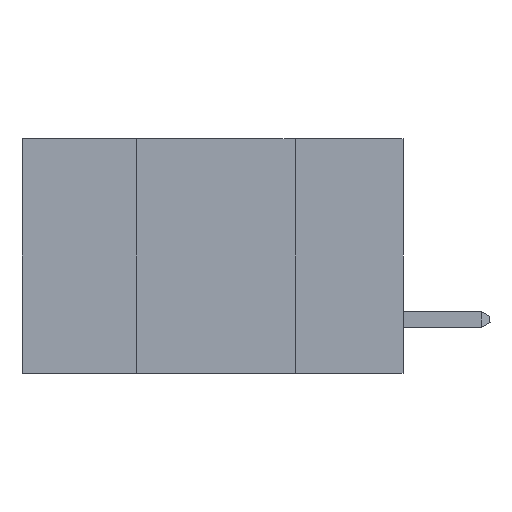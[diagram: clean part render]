
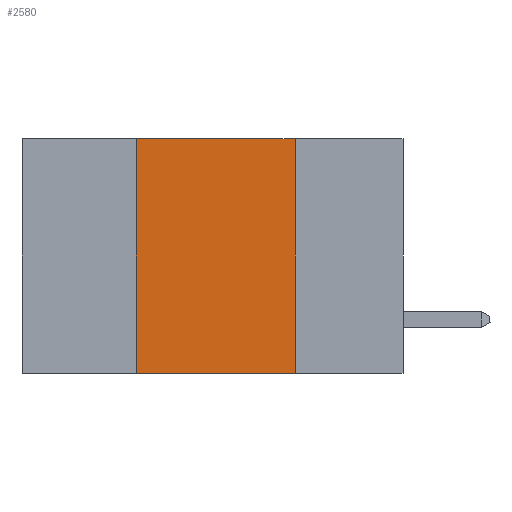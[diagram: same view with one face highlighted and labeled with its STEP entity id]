
A CAD part, left-side view. The second image highlights one B-rep face of the part: STEP entity #2580.
In plain terms, the highlighted planar face has unit normal (-1, 0, 0).
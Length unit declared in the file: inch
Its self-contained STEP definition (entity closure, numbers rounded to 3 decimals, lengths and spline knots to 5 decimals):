
#1754 = VERTEX_POINT ( 'NONE', #9888 ) ;
#2580 = ADVANCED_FACE ( 'NONE', ( #19786 ), #27750, .F. ) ;
#2932 = LINE ( 'NONE', #18165, #22426 ) ;
#3653 = VECTOR ( 'NONE', #15834, 39.37008 ) ;
#4585 = DIRECTION ( 'NONE',  ( 0., -1., 0. ) ) ;
#4915 = ORIENTED_EDGE ( 'NONE', *, *, #22747, .F. ) ;
#6339 = VECTOR ( 'NONE', #30227, 39.37008 ) ;
#6555 = DIRECTION ( 'NONE',  ( 0., 0., -1. ) ) ;
#7810 = VERTEX_POINT ( 'NONE', #13854 ) ;
#8542 = DIRECTION ( 'NONE',  ( 0., 0., -1. ) ) ;
#8993 = EDGE_CURVE ( 'NONE', #1754, #7810, #19087, .T. ) ;
#9042 = CARTESIAN_POINT ( 'NONE',  ( 0., 0.6, 0. ) ) ;
#9888 = CARTESIAN_POINT ( 'NONE',  ( 0., 0.42, 0. ) ) ;
#13569 = DIRECTION ( 'NONE',  ( 1., 0., 0. ) ) ;
#13854 = CARTESIAN_POINT ( 'NONE',  ( 0., 0.17, 0. ) ) ;
#15087 = LINE ( 'NONE', #27662, #3653 ) ;
#15834 = DIRECTION ( 'NONE',  ( 0., -1., 0. ) ) ;
#17259 = EDGE_CURVE ( 'NONE', #28613, #25607, #15087, .T. ) ;
#17605 = VECTOR ( 'NONE', #4585, 39.37008 ) ;
#18165 = CARTESIAN_POINT ( 'NONE',  ( 0., 0.17, 0. ) ) ;
#18462 = CARTESIAN_POINT ( 'NONE',  ( 0., 0.6, 0. ) ) ;
#18839 = LINE ( 'NONE', #25690, #6339 ) ;
#19087 = LINE ( 'NONE', #18462, #17605 ) ;
#19786 = FACE_OUTER_BOUND ( 'NONE', #27410, .T. ) ;
#20656 = EDGE_CURVE ( 'NONE', #28613, #1754, #18839, .T. ) ;
#20707 = ORIENTED_EDGE ( 'NONE', *, *, #20656, .F. ) ;
#22426 = VECTOR ( 'NONE', #8542, 39.37008 ) ;
#22739 = AXIS2_PLACEMENT_3D ( 'NONE', #9042, #13569, #6555 ) ;
#22747 = EDGE_CURVE ( 'NONE', #7810, #25607, #2932, .T. ) ;
#23210 = ORIENTED_EDGE ( 'NONE', *, *, #17259, .T. ) ;
#25607 = VERTEX_POINT ( 'NONE', #28980 ) ;
#25690 = CARTESIAN_POINT ( 'NONE',  ( 0., 0.42, 0. ) ) ;
#25906 = CARTESIAN_POINT ( 'NONE',  ( 0., 0.42, -0.37 ) ) ;
#27150 = ORIENTED_EDGE ( 'NONE', *, *, #8993, .F. ) ;
#27410 = EDGE_LOOP ( 'NONE', ( #4915, #27150, #20707, #23210 ) ) ;
#27662 = CARTESIAN_POINT ( 'NONE',  ( 0., 0.6, -0.37 ) ) ;
#27750 = PLANE ( 'NONE',  #22739 ) ;
#28613 = VERTEX_POINT ( 'NONE', #25906 ) ;
#28980 = CARTESIAN_POINT ( 'NONE',  ( 0., 0.17, -0.37 ) ) ;
#30227 = DIRECTION ( 'NONE',  ( 0., 0., 1. ) ) ;
